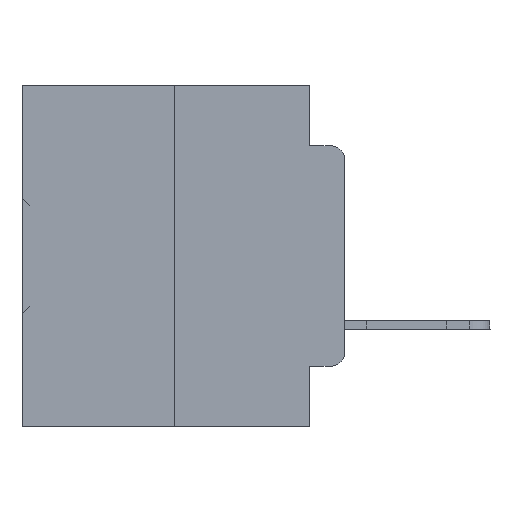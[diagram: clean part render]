
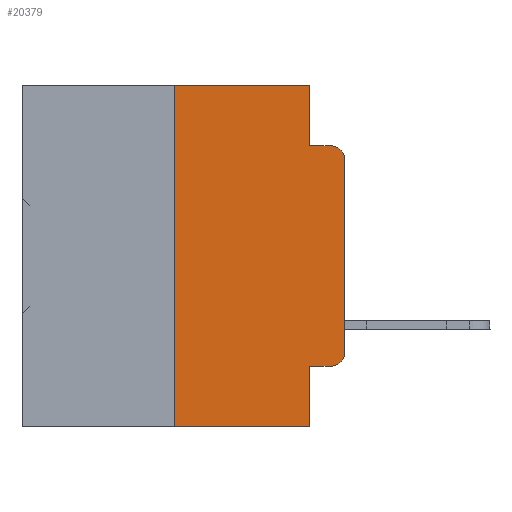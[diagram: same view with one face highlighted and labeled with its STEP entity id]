
A CAD part, left-side view. The second image highlights one B-rep face of the part: STEP entity #20379.
In plain terms, the highlighted planar face has unit normal (-1, 0, 0).
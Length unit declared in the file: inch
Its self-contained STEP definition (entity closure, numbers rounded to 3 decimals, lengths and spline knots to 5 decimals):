
#740 = VECTOR ( 'NONE', #26539, 39.37008 ) ;
#1156 = VERTEX_POINT ( 'NONE', #25447 ) ;
#1687 = AXIS2_PLACEMENT_3D ( 'NONE', #11143, #17185, #28903 ) ;
#2609 = DIRECTION ( 'NONE',  ( 0., 0., -1. ) ) ;
#2791 = EDGE_CURVE ( 'NONE', #1156, #29132, #18336, .T. ) ;
#3049 = VECTOR ( 'NONE', #20105, 39.37008 ) ;
#3114 = DIRECTION ( 'NONE',  ( 0., 0., -1. ) ) ;
#3377 = VECTOR ( 'NONE', #2609, 39.37008 ) ;
#3531 = VERTEX_POINT ( 'NONE', #35817 ) ;
#3752 = CARTESIAN_POINT ( 'NONE',  ( 0., 0., -0.3915 ) ) ;
#3881 = ORIENTED_EDGE ( 'NONE', *, *, #6871, .T. ) ;
#3996 = ORIENTED_EDGE ( 'NONE', *, *, #18264, .T. ) ;
#4019 = VECTOR ( 'NONE', #18804, 39.37008 ) ;
#4072 = EDGE_CURVE ( 'NONE', #28393, #5817, #15472, .T. ) ;
#5779 = CARTESIAN_POINT ( 'NONE',  ( 0., 0.051, -0.4115 ) ) ;
#5817 = VERTEX_POINT ( 'NONE', #22514 ) ;
#6164 = CARTESIAN_POINT ( 'NONE',  ( 0., 0.25, 0. ) ) ;
#6288 = ORIENTED_EDGE ( 'NONE', *, *, #2791, .F. ) ;
#6392 = ORIENTED_EDGE ( 'NONE', *, *, #32384, .F. ) ;
#6527 = CARTESIAN_POINT ( 'NONE',  ( 0., 0.02, -0.3915 ) ) ;
#6589 = ORIENTED_EDGE ( 'NONE', *, *, #4072, .F. ) ;
#6659 = AXIS2_PLACEMENT_3D ( 'NONE', #6527, #15258, #3114 ) ;
#6871 = EDGE_CURVE ( 'NONE', #37496, #26566, #12885, .T. ) ;
#6874 = LINE ( 'NONE', #5779, #740 ) ;
#6928 = EDGE_CURVE ( 'NONE', #26566, #3531, #20869, .T. ) ;
#7591 = DIRECTION ( 'NONE',  ( 0., -1., 0. ) ) ;
#11143 = CARTESIAN_POINT ( 'NONE',  ( 0., 0.473, 0. ) ) ;
#11399 = CARTESIAN_POINT ( 'NONE',  ( 0., 0.051, 0. ) ) ;
#12140 = DIRECTION ( 'NONE',  ( 0., 0., 1. ) ) ;
#12146 = CARTESIAN_POINT ( 'NONE',  ( 0., 0.25, -0.5 ) ) ;
#12395 = ORIENTED_EDGE ( 'NONE', *, *, #6928, .T. ) ;
#12885 = CIRCLE ( 'NONE', #6659, 0.02 ) ;
#13169 = EDGE_LOOP ( 'NONE', ( #12395, #3996, #6392, #6589, #22285, #24841, #32941, #6288, #21788, #3881 ) ) ;
#13302 = CARTESIAN_POINT ( 'NONE',  ( 0., 0.473, 0. ) ) ;
#13767 = VERTEX_POINT ( 'NONE', #37530 ) ;
#13894 = DIRECTION ( 'NONE',  ( -1., 0., 0. ) ) ;
#14362 = CARTESIAN_POINT ( 'NONE',  ( 0., 0.051, 0. ) ) ;
#15157 = CARTESIAN_POINT ( 'NONE',  ( 0., 0.02, -0.0885 ) ) ;
#15258 = DIRECTION ( 'NONE',  ( -1., 0., 0. ) ) ;
#15472 = LINE ( 'NONE', #38617, #26693 ) ;
#16474 = CARTESIAN_POINT ( 'NONE',  ( 0., 0.02, -0.4115 ) ) ;
#16534 = CIRCLE ( 'NONE', #25448, 0.02 ) ;
#17185 = DIRECTION ( 'NONE',  ( 1., 0., 0. ) ) ;
#17389 = VERTEX_POINT ( 'NONE', #12146 ) ;
#18264 = EDGE_CURVE ( 'NONE', #3531, #34360, #16534, .T. ) ;
#18336 = LINE ( 'NONE', #14362, #3377 ) ;
#18804 = DIRECTION ( 'NONE',  ( 0., 0., 1. ) ) ;
#19968 = EDGE_CURVE ( 'NONE', #17389, #29132, #36346, .T. ) ;
#20105 = DIRECTION ( 'NONE',  ( 0., -1., 0. ) ) ;
#20351 = LINE ( 'NONE', #37887, #3049 ) ;
#20379 = ADVANCED_FACE ( 'NONE', ( #26092 ), #20845, .F. ) ;
#20845 = PLANE ( 'NONE',  #1687 ) ;
#20869 = LINE ( 'NONE', #22701, #4019 ) ;
#21788 = ORIENTED_EDGE ( 'NONE', *, *, #37689, .T. ) ;
#22285 = ORIENTED_EDGE ( 'NONE', *, *, #22594, .F. ) ;
#22514 = CARTESIAN_POINT ( 'NONE',  ( 0., 0.051, -0.0885 ) ) ;
#22594 = EDGE_CURVE ( 'NONE', #13767, #28393, #28731, .T. ) ;
#22701 = CARTESIAN_POINT ( 'NONE',  ( 0., 0., 0. ) ) ;
#23561 = LINE ( 'NONE', #6164, #36567 ) ;
#24841 = ORIENTED_EDGE ( 'NONE', *, *, #36317, .F. ) ;
#25447 = CARTESIAN_POINT ( 'NONE',  ( 0., 0.051, -0.4115 ) ) ;
#25448 = AXIS2_PLACEMENT_3D ( 'NONE', #34351, #13894, #34754 ) ;
#26092 = FACE_OUTER_BOUND ( 'NONE', #13169, .T. ) ;
#26539 = DIRECTION ( 'NONE',  ( 0., -1., 0. ) ) ;
#26566 = VERTEX_POINT ( 'NONE', #3752 ) ;
#26693 = VECTOR ( 'NONE', #38491, 39.37008 ) ;
#27273 = DIRECTION ( 'NONE',  ( 0., -1., 0. ) ) ;
#28393 = VERTEX_POINT ( 'NONE', #11399 ) ;
#28731 = LINE ( 'NONE', #13302, #36643 ) ;
#28903 = DIRECTION ( 'NONE',  ( 0., 0., -1. ) ) ;
#29132 = VERTEX_POINT ( 'NONE', #33365 ) ;
#32384 = EDGE_CURVE ( 'NONE', #5817, #34360, #20351, .T. ) ;
#32941 = ORIENTED_EDGE ( 'NONE', *, *, #19968, .T. ) ;
#33365 = CARTESIAN_POINT ( 'NONE',  ( 0., 0.051, -0.5 ) ) ;
#34351 = CARTESIAN_POINT ( 'NONE',  ( 0., 0.02, -0.1085 ) ) ;
#34360 = VERTEX_POINT ( 'NONE', #15157 ) ;
#34754 = DIRECTION ( 'NONE',  ( 0., 0., -1. ) ) ;
#35817 = CARTESIAN_POINT ( 'NONE',  ( 0., 0., -0.1085 ) ) ;
#35940 = CARTESIAN_POINT ( 'NONE',  ( 0., 0.473, -0.5 ) ) ;
#36317 = EDGE_CURVE ( 'NONE', #17389, #13767, #23561, .T. ) ;
#36346 = LINE ( 'NONE', #35940, #38183 ) ;
#36567 = VECTOR ( 'NONE', #12140, 39.37008 ) ;
#36643 = VECTOR ( 'NONE', #7591, 39.37008 ) ;
#37496 = VERTEX_POINT ( 'NONE', #16474 ) ;
#37530 = CARTESIAN_POINT ( 'NONE',  ( 0., 0.25, 0. ) ) ;
#37689 = EDGE_CURVE ( 'NONE', #1156, #37496, #6874, .T. ) ;
#37887 = CARTESIAN_POINT ( 'NONE',  ( 0., 0.051, -0.0885 ) ) ;
#38183 = VECTOR ( 'NONE', #27273, 39.37008 ) ;
#38491 = DIRECTION ( 'NONE',  ( 0., 0., -1. ) ) ;
#38617 = CARTESIAN_POINT ( 'NONE',  ( 0., 0.051, 0. ) ) ;
